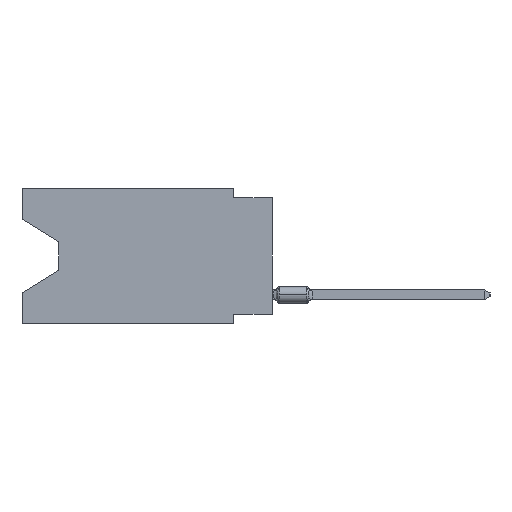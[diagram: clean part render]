
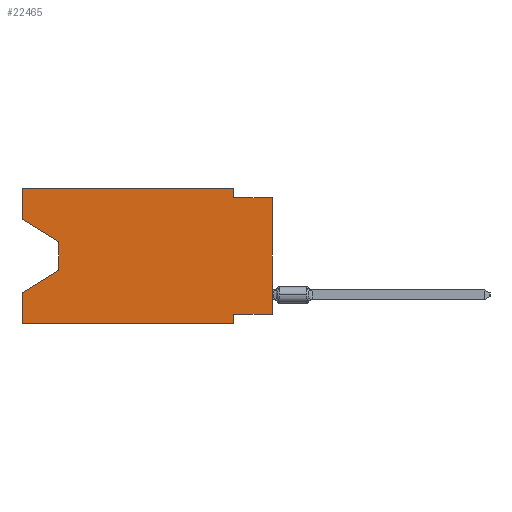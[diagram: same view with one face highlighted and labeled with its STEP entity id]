
A CAD part, left-side view. The second image highlights one B-rep face of the part: STEP entity #22465.
In plain terms, the highlighted planar face has unit normal (-1, 0, 0).
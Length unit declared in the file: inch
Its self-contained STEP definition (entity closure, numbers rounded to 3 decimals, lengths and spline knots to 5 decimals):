
#82 = PLANE ( 'NONE',  #6422 ) ;
#787 = CARTESIAN_POINT ( 'NONE',  ( 0., 0., -0.325 ) ) ;
#809 = DIRECTION ( 'NONE',  ( 0., 0., -1. ) ) ;
#1062 = CARTESIAN_POINT ( 'NONE',  ( 0., 0.55, -0.138 ) ) ;
#1623 = CARTESIAN_POINT ( 'NONE',  ( 0., 0., -0.325 ) ) ;
#1966 = VERTEX_POINT ( 'NONE', #44852 ) ;
#2078 = LINE ( 'NONE', #40032, #9812 ) ;
#2470 = ORIENTED_EDGE ( 'NONE', *, *, #39957, .F. ) ;
#2919 = EDGE_CURVE ( 'NONE', #24814, #28209, #4954, .T. ) ;
#3214 = CARTESIAN_POINT ( 'NONE',  ( 0., 0.645, -0.35 ) ) ;
#3738 = DIRECTION ( 'NONE',  ( 0., 0., 1. ) ) ;
#4053 = DIRECTION ( 'NONE',  ( 0., 0., -1. ) ) ;
#4273 = CARTESIAN_POINT ( 'NONE',  ( 0., 0.1, 0. ) ) ;
#4306 = DIRECTION ( 'NONE',  ( 1., 0., 0. ) ) ;
#4481 = ORIENTED_EDGE ( 'NONE', *, *, #2919, .T. ) ;
#4530 = ORIENTED_EDGE ( 'NONE', *, *, #28963, .T. ) ;
#4954 = LINE ( 'NONE', #16847, #9040 ) ;
#6422 = AXIS2_PLACEMENT_3D ( 'NONE', #19694, #4306, #4053 ) ;
#6718 = VECTOR ( 'NONE', #12451, 39.37008 ) ;
#7397 = DIRECTION ( 'NONE',  ( 0., -1., 0. ) ) ;
#7555 = CARTESIAN_POINT ( 'NONE',  ( 0., 0.645, 0. ) ) ;
#7983 = DIRECTION ( 'NONE',  ( 0., 0.855, -0.519 ) ) ;
#9040 = VECTOR ( 'NONE', #20093, 39.37008 ) ;
#9795 = VERTEX_POINT ( 'NONE', #13535 ) ;
#9812 = VECTOR ( 'NONE', #14209, 39.37008 ) ;
#9972 = VECTOR ( 'NONE', #7397, 39.37008 ) ;
#10198 = EDGE_CURVE ( 'NONE', #22765, #1966, #2078, .T. ) ;
#10244 = ORIENTED_EDGE ( 'NONE', *, *, #10542, .F. ) ;
#10542 = EDGE_CURVE ( 'NONE', #34432, #11733, #19657, .T. ) ;
#11733 = VERTEX_POINT ( 'NONE', #30977 ) ;
#11884 = ORIENTED_EDGE ( 'NONE', *, *, #37476, .T. ) ;
#12451 = DIRECTION ( 'NONE',  ( 0., 0., -1. ) ) ;
#12686 = CARTESIAN_POINT ( 'NONE',  ( 0., 0.55, -0.212 ) ) ;
#13535 = CARTESIAN_POINT ( 'NONE',  ( 0., 0.55, -0.212 ) ) ;
#14209 = DIRECTION ( 'NONE',  ( 0., -1., 0. ) ) ;
#15639 = VERTEX_POINT ( 'NONE', #35198 ) ;
#15740 = ORIENTED_EDGE ( 'NONE', *, *, #31640, .T. ) ;
#15921 = DIRECTION ( 'NONE',  ( 0., 1., 0. ) ) ;
#16189 = LINE ( 'NONE', #1062, #19605 ) ;
#16847 = CARTESIAN_POINT ( 'NONE',  ( 0., 0.645, -0.08025 ) ) ;
#17367 = VECTOR ( 'NONE', #15921, 39.37008 ) ;
#17426 = VECTOR ( 'NONE', #7983, 39.37008 ) ;
#17560 = VECTOR ( 'NONE', #30965, 39.37008 ) ;
#18405 = VERTEX_POINT ( 'NONE', #7555 ) ;
#18444 = CARTESIAN_POINT ( 'NONE',  ( 0., 0., 0. ) ) ;
#19605 = VECTOR ( 'NONE', #809, 39.37008 ) ;
#19657 = LINE ( 'NONE', #787, #17367 ) ;
#19694 = CARTESIAN_POINT ( 'NONE',  ( 0., 0.645, 0. ) ) ;
#20093 = DIRECTION ( 'NONE',  ( 0., -0.855, -0.519 ) ) ;
#20334 = EDGE_LOOP ( 'NONE', ( #4481, #21537, #4530, #40981, #15740, #47567, #10244, #11884, #22532, #43158, #30750, #2470 ) ) ;
#21390 = CARTESIAN_POINT ( 'NONE',  ( 0., 0.1, 0. ) ) ;
#21537 = ORIENTED_EDGE ( 'NONE', *, *, #48456, .T. ) ;
#21965 = CARTESIAN_POINT ( 'NONE',  ( 0., 0.55, -0.138 ) ) ;
#22465 = ADVANCED_FACE ( 'NONE', ( #30365 ), #82, .F. ) ;
#22532 = ORIENTED_EDGE ( 'NONE', *, *, #10198, .F. ) ;
#22765 = VERTEX_POINT ( 'NONE', #36103 ) ;
#23868 = LINE ( 'NONE', #4273, #6718 ) ;
#24736 = VECTOR ( 'NONE', #33232, 39.37008 ) ;
#24814 = VERTEX_POINT ( 'NONE', #47696 ) ;
#25909 = VERTEX_POINT ( 'NONE', #21390 ) ;
#28209 = VERTEX_POINT ( 'NONE', #21965 ) ;
#28963 = EDGE_CURVE ( 'NONE', #9795, #30296, #46439, .T. ) ;
#29294 = EDGE_CURVE ( 'NONE', #11733, #36605, #31432, .T. ) ;
#30296 = VERTEX_POINT ( 'NONE', #42452 ) ;
#30365 = FACE_OUTER_BOUND ( 'NONE', #20334, .T. ) ;
#30451 = CARTESIAN_POINT ( 'NONE',  ( 0., 0.645, 0. ) ) ;
#30719 = CARTESIAN_POINT ( 'NONE',  ( 0., 0.645, 0. ) ) ;
#30750 = ORIENTED_EDGE ( 'NONE', *, *, #47098, .F. ) ;
#30965 = DIRECTION ( 'NONE',  ( 0., 0., 1. ) ) ;
#30977 = CARTESIAN_POINT ( 'NONE',  ( 0., 0.1, -0.325 ) ) ;
#31432 = LINE ( 'NONE', #35642, #41226 ) ;
#31640 = EDGE_CURVE ( 'NONE', #15639, #36605, #33726, .T. ) ;
#33232 = DIRECTION ( 'NONE',  ( 0., -1., 0. ) ) ;
#33451 = LINE ( 'NONE', #30451, #9972 ) ;
#33682 = CARTESIAN_POINT ( 'NONE',  ( 0., 0.1, -0.35 ) ) ;
#33726 = LINE ( 'NONE', #3214, #24736 ) ;
#34432 = VERTEX_POINT ( 'NONE', #1623 ) ;
#35198 = CARTESIAN_POINT ( 'NONE',  ( 0., 0.645, -0.35 ) ) ;
#35642 = CARTESIAN_POINT ( 'NONE',  ( 0., 0.1, -0.35 ) ) ;
#36103 = CARTESIAN_POINT ( 'NONE',  ( 0., 0.1, -0.025 ) ) ;
#36460 = LINE ( 'NONE', #30719, #17560 ) ;
#36605 = VERTEX_POINT ( 'NONE', #33682 ) ;
#37476 = EDGE_CURVE ( 'NONE', #34432, #1966, #44742, .T. ) ;
#37551 = EDGE_CURVE ( 'NONE', #25909, #22765, #23868, .T. ) ;
#37739 = CARTESIAN_POINT ( 'NONE',  ( 0., 0.645, 0. ) ) ;
#39957 = EDGE_CURVE ( 'NONE', #24814, #18405, #41465, .T. ) ;
#40017 = VECTOR ( 'NONE', #45216, 39.37008 ) ;
#40032 = CARTESIAN_POINT ( 'NONE',  ( 0., 0., -0.025 ) ) ;
#40391 = VECTOR ( 'NONE', #3738, 39.37008 ) ;
#40981 = ORIENTED_EDGE ( 'NONE', *, *, #41451, .F. ) ;
#41226 = VECTOR ( 'NONE', #42835, 39.37008 ) ;
#41451 = EDGE_CURVE ( 'NONE', #15639, #30296, #36460, .T. ) ;
#41465 = LINE ( 'NONE', #37739, #40391 ) ;
#42452 = CARTESIAN_POINT ( 'NONE',  ( 0., 0.645, -0.26975 ) ) ;
#42835 = DIRECTION ( 'NONE',  ( 0., 0., -1. ) ) ;
#43158 = ORIENTED_EDGE ( 'NONE', *, *, #37551, .F. ) ;
#44742 = LINE ( 'NONE', #18444, #40017 ) ;
#44852 = CARTESIAN_POINT ( 'NONE',  ( 0., 0., -0.025 ) ) ;
#45216 = DIRECTION ( 'NONE',  ( 0., 0., 1. ) ) ;
#46439 = LINE ( 'NONE', #12686, #17426 ) ;
#47098 = EDGE_CURVE ( 'NONE', #18405, #25909, #33451, .T. ) ;
#47567 = ORIENTED_EDGE ( 'NONE', *, *, #29294, .F. ) ;
#47696 = CARTESIAN_POINT ( 'NONE',  ( 0., 0.645, -0.08025 ) ) ;
#48456 = EDGE_CURVE ( 'NONE', #28209, #9795, #16189, .T. ) ;
